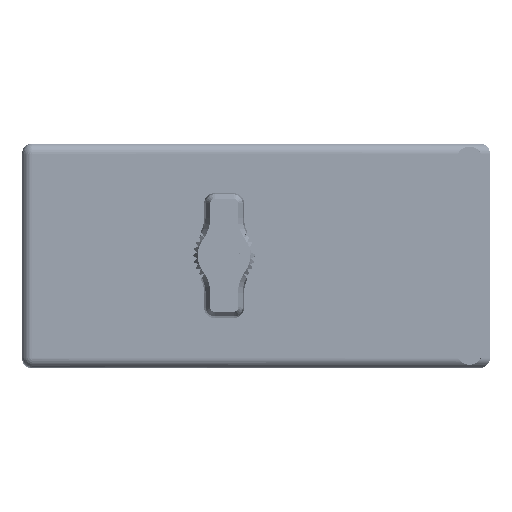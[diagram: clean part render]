
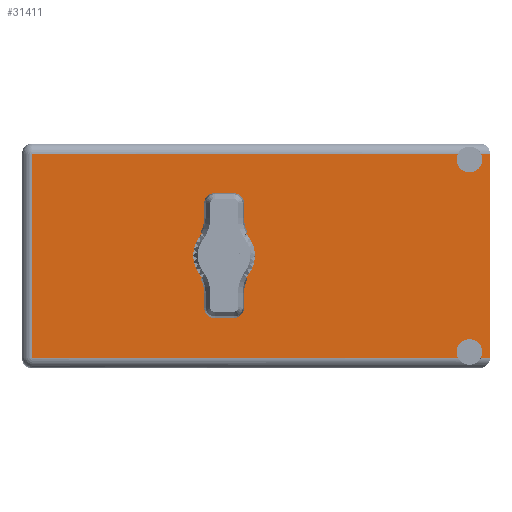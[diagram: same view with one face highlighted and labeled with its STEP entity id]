
A CAD part, top view. The second image highlights one B-rep face of the part: STEP entity #31411.
In plain terms, the highlighted face is planar.
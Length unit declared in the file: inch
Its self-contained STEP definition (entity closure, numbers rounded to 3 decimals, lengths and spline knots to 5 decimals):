
#2556 = VERTEX_POINT ( 'NONE', #42901 ) ;
#2688 = CARTESIAN_POINT ( 'NONE',  ( 1.6725, 1.93, 0.656 ) ) ;
#2844 = EDGE_LOOP ( 'NONE', ( #72236, #31053 ) ) ;
#4290 = LINE ( 'NONE', #56509, #9405 ) ;
#4739 = ORIENTED_EDGE ( 'NONE', *, *, #20958, .F. ) ;
#5285 = DIRECTION ( 'NONE',  ( 0., 0., 1. ) ) ;
#5374 = CARTESIAN_POINT ( 'NONE',  ( 0., 1.93, -0.17 ) ) ;
#5839 = DIRECTION ( 'NONE',  ( 0., 1., 0. ) ) ;
#6191 = DIRECTION ( 'NONE',  ( 0., 0., 1. ) ) ;
#6333 = DIRECTION ( 'NONE',  ( 0., 1., 0. ) ) ;
#9405 = VECTOR ( 'NONE', #94303, 39.37008 ) ;
#11636 = ORIENTED_EDGE ( 'NONE', *, *, #29747, .F. ) ;
#11769 = AXIS2_PLACEMENT_3D ( 'NONE', #71450, #47651, #55125 ) ;
#16995 = CARTESIAN_POINT ( 'NONE',  ( -1.3075, 1.93, -0.695 ) ) ;
#20958 = EDGE_CURVE ( 'NONE', #55988, #26450, #71165, .T. ) ;
#21318 = ORIENTED_EDGE ( 'NONE', *, *, #103726, .T. ) ;
#21993 = VERTEX_POINT ( 'NONE', #94121 ) ;
#22753 = EDGE_CURVE ( 'NONE', #41154, #26450, #42146, .T. ) ;
#23414 = CIRCLE ( 'NONE', #11769, 0.0875 ) ;
#23586 = DIRECTION ( 'NONE',  ( -1., 0., 0. ) ) ;
#23699 = CARTESIAN_POINT ( 'NONE',  ( -1.3075, 1.93, -0.765 ) ) ;
#24903 = VERTEX_POINT ( 'NONE', #30409 ) ;
#26450 = VERTEX_POINT ( 'NONE', #68147 ) ;
#26563 = DIRECTION ( 'NONE',  ( 0., 1., 0. ) ) ;
#26627 = CARTESIAN_POINT ( 'NONE',  ( 1.6725, 1.93, -0.5685 ) ) ;
#28447 = ORIENTED_EDGE ( 'NONE', *, *, #63695, .T. ) ;
#29747 = EDGE_CURVE ( 'NONE', #84631, #33679, #23414, .T. ) ;
#30409 = CARTESIAN_POINT ( 'NONE',  ( 1.59417, 1.93, -0.695 ) ) ;
#31053 = ORIENTED_EDGE ( 'NONE', *, *, #105225, .F. ) ;
#31315 = VECTOR ( 'NONE', #80684, 39.37008 ) ;
#31411 = ADVANCED_FACE ( 'NONE', ( #53735, #31990 ), #88404, .T. ) ;
#31990 = FACE_OUTER_BOUND ( 'NONE', #92035, .T. ) ;
#32707 = VECTOR ( 'NONE', #98770, 39.37008 ) ;
#33055 = ORIENTED_EDGE ( 'NONE', *, *, #67235, .T. ) ;
#33679 = VERTEX_POINT ( 'NONE', #66918 ) ;
#34288 = CARTESIAN_POINT ( 'NONE',  ( 1.75083, 1.93, 0.695 ) ) ;
#35937 = VERTEX_POINT ( 'NONE', #72110 ) ;
#37155 = LINE ( 'NONE', #102848, #42225 ) ;
#38968 = CARTESIAN_POINT ( 'NONE',  ( 0., 1.93, 0. ) ) ;
#39625 = DIRECTION ( 'NONE',  ( 0., 1., 0. ) ) ;
#40336 = VERTEX_POINT ( 'NONE', #34288 ) ;
#40510 = LINE ( 'NONE', #59840, #74932 ) ;
#41154 = VERTEX_POINT ( 'NONE', #82523 ) ;
#41752 = CARTESIAN_POINT ( 'NONE',  ( 1.8125, 1.93, 0.695 ) ) ;
#41979 = AXIS2_PLACEMENT_3D ( 'NONE', #95785, #6333, #5285 ) ;
#42146 = LINE ( 'NONE', #97506, #58699 ) ;
#42225 = VECTOR ( 'NONE', #95054, 39.37008 ) ;
#42901 = CARTESIAN_POINT ( 'NONE',  ( 0., 1.93, 0.17 ) ) ;
#42934 = EDGE_CURVE ( 'NONE', #2556, #82402, #96845, .T. ) ;
#43266 = EDGE_CURVE ( 'NONE', #40336, #84631, #48332, .T. ) ;
#45405 = AXIS2_PLACEMENT_3D ( 'NONE', #92573, #68664, #52720 ) ;
#46183 = DIRECTION ( 'NONE',  ( 0., 1., 0. ) ) ;
#47651 = DIRECTION ( 'NONE',  ( 0., 1., 0. ) ) ;
#48332 = CIRCLE ( 'NONE', #100691, 0.0875 ) ;
#48551 = ORIENTED_EDGE ( 'NONE', *, *, #22753, .T. ) ;
#48602 = EDGE_CURVE ( 'NONE', #24903, #55988, #74947, .T. ) ;
#52720 = DIRECTION ( 'NONE',  ( 0., 0., 1. ) ) ;
#53735 = FACE_BOUND ( 'NONE', #2844, .T. ) ;
#55125 = DIRECTION ( 'NONE',  ( 0., 0., 1. ) ) ;
#55988 = VERTEX_POINT ( 'NONE', #26627 ) ;
#56509 = CARTESIAN_POINT ( 'NONE',  ( 1.8125, 1.93, 0.695 ) ) ;
#58093 = AXIS2_PLACEMENT_3D ( 'NONE', #78893, #46183, #96328 ) ;
#58699 = VECTOR ( 'NONE', #89958, 39.37008 ) ;
#59840 = CARTESIAN_POINT ( 'NONE',  ( 1.8125, 1.93, 0.765 ) ) ;
#62838 = EDGE_CURVE ( 'NONE', #90382, #21993, #70754, .T. ) ;
#63116 = ORIENTED_EDGE ( 'NONE', *, *, #76670, .F. ) ;
#63695 = EDGE_CURVE ( 'NONE', #21993, #33679, #4290, .T. ) ;
#66918 = CARTESIAN_POINT ( 'NONE',  ( 1.59417, 1.93, 0.695 ) ) ;
#67235 = EDGE_CURVE ( 'NONE', #24903, #90382, #37155, .T. ) ;
#68147 = CARTESIAN_POINT ( 'NONE',  ( 1.75083, 1.93, -0.695 ) ) ;
#68664 = DIRECTION ( 'NONE',  ( 0., 1., 0. ) ) ;
#70754 = LINE ( 'NONE', #23699, #31315 ) ;
#71165 = CIRCLE ( 'NONE', #45405, 0.0875 ) ;
#71450 = CARTESIAN_POINT ( 'NONE',  ( 1.6725, 1.93, 0.656 ) ) ;
#72110 = CARTESIAN_POINT ( 'NONE',  ( 1.8125, 1.93, 0.695 ) ) ;
#72236 = ORIENTED_EDGE ( 'NONE', *, *, #42934, .F. ) ;
#74530 = CIRCLE ( 'NONE', #82088, 0.17 ) ;
#74932 = VECTOR ( 'NONE', #92611, 39.37008 ) ;
#74947 = CIRCLE ( 'NONE', #58093, 0.0875 ) ;
#75359 = DIRECTION ( 'NONE',  ( 0., 0., 1. ) ) ;
#76041 = LINE ( 'NONE', #41752, #32707 ) ;
#76670 = EDGE_CURVE ( 'NONE', #41154, #35937, #40510, .T. ) ;
#78893 = CARTESIAN_POINT ( 'NONE',  ( 1.6725, 1.93, -0.656 ) ) ;
#79870 = CARTESIAN_POINT ( 'NONE',  ( -1.3775, 1.93, -0.765 ) ) ;
#80684 = DIRECTION ( 'NONE',  ( 0., 0., 1. ) ) ;
#82088 = AXIS2_PLACEMENT_3D ( 'NONE', #38968, #5839, #6191 ) ;
#82402 = VERTEX_POINT ( 'NONE', #5374 ) ;
#82523 = CARTESIAN_POINT ( 'NONE',  ( 1.8125, 1.93, -0.695 ) ) ;
#84631 = VERTEX_POINT ( 'NONE', #92936 ) ;
#88341 = AXIS2_PLACEMENT_3D ( 'NONE', #79870, #39625, #23586 ) ;
#88404 = PLANE ( 'NONE',  #88341 ) ;
#89958 = DIRECTION ( 'NONE',  ( -1., 0., 0. ) ) ;
#90382 = VERTEX_POINT ( 'NONE', #16995 ) ;
#92035 = EDGE_LOOP ( 'NONE', ( #28447, #11636, #101241, #21318, #63116, #48551, #4739, #97679, #33055, #96251 ) ) ;
#92573 = CARTESIAN_POINT ( 'NONE',  ( 1.6725, 1.93, -0.656 ) ) ;
#92611 = DIRECTION ( 'NONE',  ( 0., 0., 1. ) ) ;
#92936 = CARTESIAN_POINT ( 'NONE',  ( 1.6725, 1.93, 0.5685 ) ) ;
#94121 = CARTESIAN_POINT ( 'NONE',  ( -1.3075, 1.93, 0.695 ) ) ;
#94303 = DIRECTION ( 'NONE',  ( 1., 0., 0. ) ) ;
#95054 = DIRECTION ( 'NONE',  ( -1., 0., 0. ) ) ;
#95785 = CARTESIAN_POINT ( 'NONE',  ( 0., 1.93, 0. ) ) ;
#96251 = ORIENTED_EDGE ( 'NONE', *, *, #62838, .T. ) ;
#96328 = DIRECTION ( 'NONE',  ( 0., 0., 1. ) ) ;
#96845 = CIRCLE ( 'NONE', #41979, 0.17 ) ;
#97506 = CARTESIAN_POINT ( 'NONE',  ( -1.3775, 1.93, -0.695 ) ) ;
#97679 = ORIENTED_EDGE ( 'NONE', *, *, #48602, .F. ) ;
#98770 = DIRECTION ( 'NONE',  ( 1., 0., 0. ) ) ;
#100691 = AXIS2_PLACEMENT_3D ( 'NONE', #2688, #26563, #75359 ) ;
#101241 = ORIENTED_EDGE ( 'NONE', *, *, #43266, .F. ) ;
#102848 = CARTESIAN_POINT ( 'NONE',  ( -1.3775, 1.93, -0.695 ) ) ;
#103726 = EDGE_CURVE ( 'NONE', #40336, #35937, #76041, .T. ) ;
#105225 = EDGE_CURVE ( 'NONE', #82402, #2556, #74530, .T. ) ;
